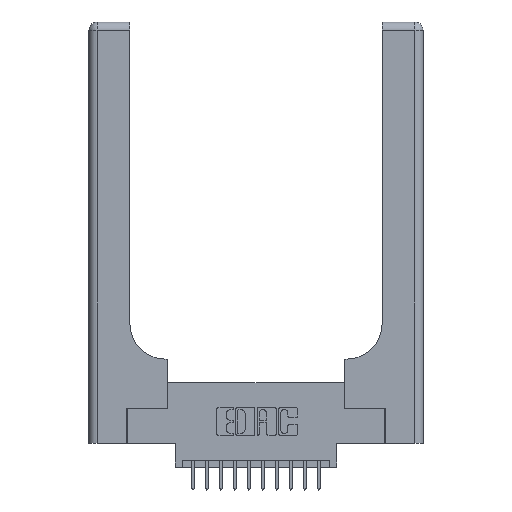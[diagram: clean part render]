
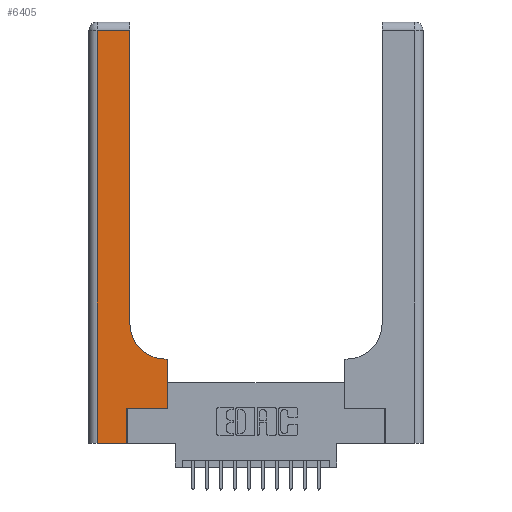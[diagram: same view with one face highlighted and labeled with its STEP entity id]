
A CAD part, top view. The second image highlights one B-rep face of the part: STEP entity #6405.
In plain terms, the highlighted planar face has unit normal (0, 0, 1).
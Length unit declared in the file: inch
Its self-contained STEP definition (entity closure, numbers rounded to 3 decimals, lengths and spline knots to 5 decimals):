
#375 = CARTESIAN_POINT ( 'NONE',  ( 0.2915, 2.94, 0.37 ) ) ;
#1220 = DIRECTION ( 'NONE',  ( -1., 0., 0. ) ) ;
#1271 = EDGE_CURVE ( 'NONE', #7589, #1408, #4483, .T. ) ;
#1400 = LINE ( 'NONE', #5396, #1614 ) ;
#1408 = VERTEX_POINT ( 'NONE', #14152 ) ;
#1420 = VECTOR ( 'NONE', #5820, 39.37008 ) ;
#1573 = VERTEX_POINT ( 'NONE', #9655 ) ;
#1614 = VECTOR ( 'NONE', #14855, 39.37008 ) ;
#1808 = CARTESIAN_POINT ( 'NONE',  ( 0.5415, 0.85, 0.37 ) ) ;
#1871 = DIRECTION ( 'NONE',  ( 0., 0., -1. ) ) ;
#2314 = VECTOR ( 'NONE', #11691, 39.37008 ) ;
#2801 = LINE ( 'NONE', #14333, #9149 ) ;
#2926 = VECTOR ( 'NONE', #7460, 39.37008 ) ;
#3750 = VERTEX_POINT ( 'NONE', #10867 ) ;
#4005 = CARTESIAN_POINT ( 'NONE',  ( 0., 3., 0.37 ) ) ;
#4164 = ORIENTED_EDGE ( 'NONE', *, *, #16810, .T. ) ;
#4223 = CARTESIAN_POINT ( 'NONE',  ( 0.5585, 0.6, 0.37 ) ) ;
#4483 = LINE ( 'NONE', #10220, #4907 ) ;
#4511 = EDGE_CURVE ( 'NONE', #1573, #16770, #17260, .T. ) ;
#4907 = VECTOR ( 'NONE', #7464, 39.37008 ) ;
#5396 = CARTESIAN_POINT ( 'NONE',  ( 0.06, 3., 0.37 ) ) ;
#5714 = ORIENTED_EDGE ( 'NONE', *, *, #9210, .T. ) ;
#5820 = DIRECTION ( 'NONE',  ( 0., 1., 0. ) ) ;
#5842 = VERTEX_POINT ( 'NONE', #6910 ) ;
#6310 = DIRECTION ( 'NONE',  ( -1., 0., 0. ) ) ;
#6405 = ADVANCED_FACE ( 'NONE', ( #14241 ), #16151, .F. ) ;
#6823 = AXIS2_PLACEMENT_3D ( 'NONE', #4005, #16202, #1220 ) ;
#6910 = CARTESIAN_POINT ( 'NONE',  ( 0.06, 2.94, 0.37 ) ) ;
#6994 = VERTEX_POINT ( 'NONE', #16829 ) ;
#7460 = DIRECTION ( 'NONE',  ( 0., 1., 0. ) ) ;
#7464 = DIRECTION ( 'NONE',  ( 1., 0., 0. ) ) ;
#7589 = VERTEX_POINT ( 'NONE', #9887 ) ;
#8455 = DIRECTION ( 'NONE',  ( 1., 0., 0. ) ) ;
#8580 = CARTESIAN_POINT ( 'NONE',  ( 0.2915, 0.85, 0.37 ) ) ;
#8736 = VERTEX_POINT ( 'NONE', #375 ) ;
#9149 = VECTOR ( 'NONE', #8455, 39.37008 ) ;
#9172 = ORIENTED_EDGE ( 'NONE', *, *, #17468, .T. ) ;
#9210 = EDGE_CURVE ( 'NONE', #5842, #7589, #1400, .T. ) ;
#9655 = CARTESIAN_POINT ( 'NONE',  ( 0.5415, 0.6, 0.37 ) ) ;
#9696 = CARTESIAN_POINT ( 'NONE',  ( 0.2915, 0.6, 0.37 ) ) ;
#9887 = CARTESIAN_POINT ( 'NONE',  ( 0.06, 0., 0.37 ) ) ;
#10115 = CARTESIAN_POINT ( 'NONE',  ( 0.269, 0., 0.37 ) ) ;
#10145 = CARTESIAN_POINT ( 'NONE',  ( 0., 2.94, 0.37 ) ) ;
#10220 = CARTESIAN_POINT ( 'NONE',  ( 0., 0., 0.37 ) ) ;
#10496 = ORIENTED_EDGE ( 'NONE', *, *, #12320, .T. ) ;
#10867 = CARTESIAN_POINT ( 'NONE',  ( 0.269, 0.25, 0.37 ) ) ;
#11017 = EDGE_LOOP ( 'NONE', ( #12137, #9172, #5714, #17063, #15447, #4164, #10496, #13789, #11804 ) ) ;
#11055 = DIRECTION ( 'NONE',  ( -1., 0., 0. ) ) ;
#11141 = VERTEX_POINT ( 'NONE', #4223 ) ;
#11180 = LINE ( 'NONE', #11471, #2926 ) ;
#11471 = CARTESIAN_POINT ( 'NONE',  ( 0.5585, 0.25, 0.37 ) ) ;
#11691 = DIRECTION ( 'NONE',  ( 0., 1., 0. ) ) ;
#11804 = ORIENTED_EDGE ( 'NONE', *, *, #4511, .T. ) ;
#11932 = EDGE_CURVE ( 'NONE', #16770, #8736, #12085, .T. ) ;
#12085 = LINE ( 'NONE', #13124, #2314 ) ;
#12137 = ORIENTED_EDGE ( 'NONE', *, *, #11932, .T. ) ;
#12320 = EDGE_CURVE ( 'NONE', #6994, #11141, #11180, .T. ) ;
#12446 = EDGE_CURVE ( 'NONE', #1408, #3750, #13960, .T. ) ;
#12567 = VECTOR ( 'NONE', #11055, 39.37008 ) ;
#12822 = AXIS2_PLACEMENT_3D ( 'NONE', #1808, #1871, #15595 ) ;
#13124 = CARTESIAN_POINT ( 'NONE',  ( 0.2915, 3., 0.37 ) ) ;
#13379 = VECTOR ( 'NONE', #6310, 39.37008 ) ;
#13789 = ORIENTED_EDGE ( 'NONE', *, *, #16736, .T. ) ;
#13960 = LINE ( 'NONE', #10115, #1420 ) ;
#14152 = CARTESIAN_POINT ( 'NONE',  ( 0.269, 0., 0.37 ) ) ;
#14241 = FACE_OUTER_BOUND ( 'NONE', #11017, .T. ) ;
#14333 = CARTESIAN_POINT ( 'NONE',  ( 0.269, 0.25, 0.37 ) ) ;
#14855 = DIRECTION ( 'NONE',  ( 0., -1., 0. ) ) ;
#15447 = ORIENTED_EDGE ( 'NONE', *, *, #12446, .T. ) ;
#15595 = DIRECTION ( 'NONE',  ( 1., 0., 0. ) ) ;
#15961 = LINE ( 'NONE', #9696, #12567 ) ;
#16151 = PLANE ( 'NONE',  #6823 ) ;
#16202 = DIRECTION ( 'NONE',  ( 0., 0., -1. ) ) ;
#16371 = LINE ( 'NONE', #10145, #13379 ) ;
#16736 = EDGE_CURVE ( 'NONE', #11141, #1573, #15961, .T. ) ;
#16770 = VERTEX_POINT ( 'NONE', #8580 ) ;
#16810 = EDGE_CURVE ( 'NONE', #3750, #6994, #2801, .T. ) ;
#16829 = CARTESIAN_POINT ( 'NONE',  ( 0.5585, 0.25, 0.37 ) ) ;
#17063 = ORIENTED_EDGE ( 'NONE', *, *, #1271, .T. ) ;
#17260 = CIRCLE ( 'NONE', #12822, 0.25 ) ;
#17468 = EDGE_CURVE ( 'NONE', #8736, #5842, #16371, .T. ) ;
